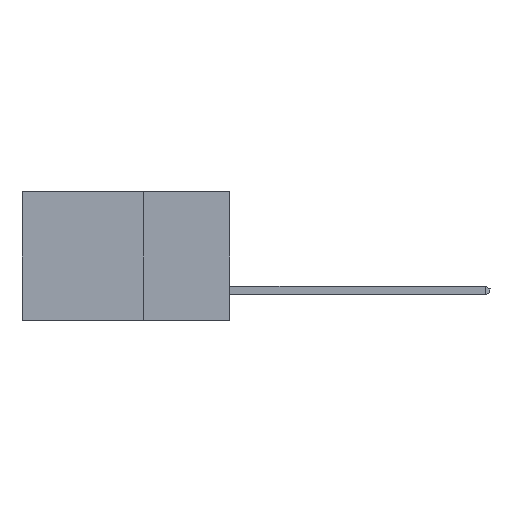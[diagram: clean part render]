
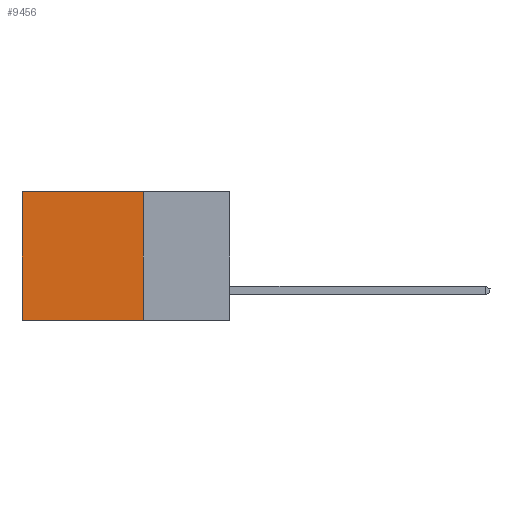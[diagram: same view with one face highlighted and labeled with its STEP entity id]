
A CAD part, left-side view. The second image highlights one B-rep face of the part: STEP entity #9456.
In plain terms, the highlighted planar face has unit normal (-1, 0, 0).
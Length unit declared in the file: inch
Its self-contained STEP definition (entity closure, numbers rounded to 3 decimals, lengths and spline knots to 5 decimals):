
#90 = CARTESIAN_POINT ( 'NONE',  ( 0.2615, 0.25, -0.37 ) ) ;
#345 = CARTESIAN_POINT ( 'NONE',  ( 0.2615, 0.25, -0.37 ) ) ;
#1071 = LINE ( 'NONE', #10316, #7514 ) ;
#1335 = DIRECTION ( 'NONE',  ( 0., 1., 0. ) ) ;
#1363 = VECTOR ( 'NONE', #4266, 39.37008 ) ;
#1402 = FACE_OUTER_BOUND ( 'NONE', #1990, .T. ) ;
#1990 = EDGE_LOOP ( 'NONE', ( #6109, #10598, #9517, #7066 ) ) ;
#2040 = VECTOR ( 'NONE', #7651, 39.37008 ) ;
#2378 = CARTESIAN_POINT ( 'NONE',  ( 0.2615, 0.25, -0.37 ) ) ;
#2979 = CARTESIAN_POINT ( 'NONE',  ( 0.2615, 0.6, -0.37 ) ) ;
#3766 = VERTEX_POINT ( 'NONE', #2378 ) ;
#3861 = DIRECTION ( 'NONE',  ( 0., 0., -1. ) ) ;
#4265 = DIRECTION ( 'NONE',  ( 0., 0., -1. ) ) ;
#4266 = DIRECTION ( 'NONE',  ( 0., 0., -1. ) ) ;
#4475 = EDGE_CURVE ( 'NONE', #7766, #7029, #7986, .T. ) ;
#4530 = EDGE_CURVE ( 'NONE', #4862, #7766, #11518, .T. ) ;
#4862 = VERTEX_POINT ( 'NONE', #12115 ) ;
#5137 = PLANE ( 'NONE',  #11294 ) ;
#5343 = VECTOR ( 'NONE', #1335, 39.37008 ) ;
#6109 = ORIENTED_EDGE ( 'NONE', *, *, #4475, .T. ) ;
#6122 = DIRECTION ( 'NONE',  ( 1., 0., 0. ) ) ;
#6493 = EDGE_CURVE ( 'NONE', #4862, #3766, #1071, .T. ) ;
#7029 = VERTEX_POINT ( 'NONE', #2979 ) ;
#7066 = ORIENTED_EDGE ( 'NONE', *, *, #4530, .T. ) ;
#7514 = VECTOR ( 'NONE', #3861, 39.37008 ) ;
#7594 = LINE ( 'NONE', #90, #2040 ) ;
#7651 = DIRECTION ( 'NONE',  ( 0., 1., 0. ) ) ;
#7766 = VERTEX_POINT ( 'NONE', #9167 ) ;
#7986 = LINE ( 'NONE', #8890, #1363 ) ;
#8374 = EDGE_CURVE ( 'NONE', #3766, #7029, #7594, .T. ) ;
#8890 = CARTESIAN_POINT ( 'NONE',  ( 0.2615, 0.6, -0.37 ) ) ;
#9167 = CARTESIAN_POINT ( 'NONE',  ( 0.2615, 0.6, 0. ) ) ;
#9456 = ADVANCED_FACE ( 'NONE', ( #1402 ), #5137, .F. ) ;
#9517 = ORIENTED_EDGE ( 'NONE', *, *, #6493, .F. ) ;
#9705 = CARTESIAN_POINT ( 'NONE',  ( 0.2615, 0.25, 0. ) ) ;
#10316 = CARTESIAN_POINT ( 'NONE',  ( 0.2615, 0.25, -0.37 ) ) ;
#10598 = ORIENTED_EDGE ( 'NONE', *, *, #8374, .F. ) ;
#11294 = AXIS2_PLACEMENT_3D ( 'NONE', #345, #6122, #4265 ) ;
#11518 = LINE ( 'NONE', #9705, #5343 ) ;
#12115 = CARTESIAN_POINT ( 'NONE',  ( 0.2615, 0.25, 0. ) ) ;
